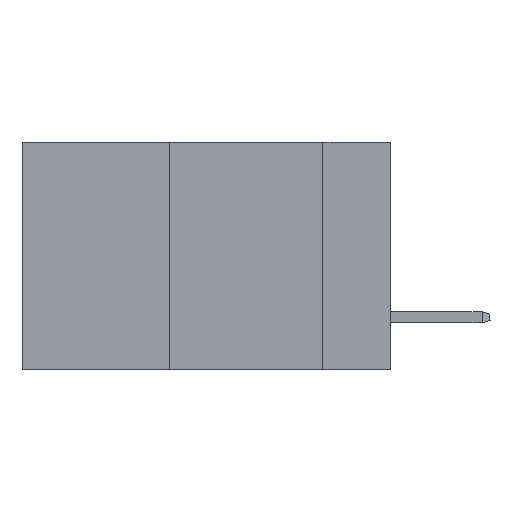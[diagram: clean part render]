
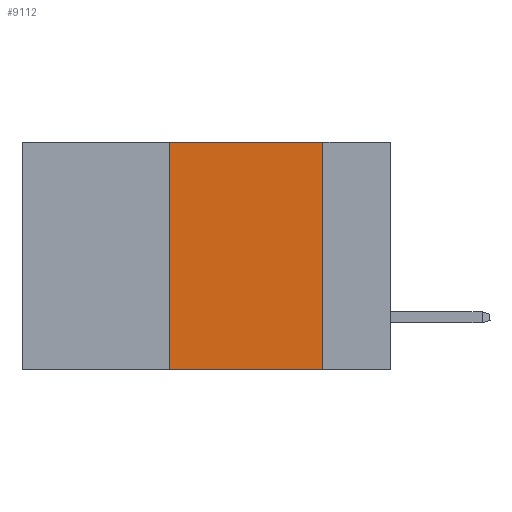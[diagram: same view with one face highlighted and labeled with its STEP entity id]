
A CAD part, left-side view. The second image highlights one B-rep face of the part: STEP entity #9112.
In plain terms, the highlighted planar face has unit normal (-1, 0, 0).
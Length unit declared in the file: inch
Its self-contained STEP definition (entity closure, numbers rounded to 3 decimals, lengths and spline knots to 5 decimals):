
#320 = CARTESIAN_POINT ( 'NONE',  ( 0., 0.11, -0.37 ) ) ;
#380 = CARTESIAN_POINT ( 'NONE',  ( 0., 0.6, -0.37 ) ) ;
#585 = ORIENTED_EDGE ( 'NONE', *, *, #3859, .F. ) ;
#831 = CARTESIAN_POINT ( 'NONE',  ( 0., 0.36, 0. ) ) ;
#1301 = EDGE_CURVE ( 'NONE', #4747, #1466, #3423, .T. ) ;
#1466 = VERTEX_POINT ( 'NONE', #320 ) ;
#3423 = LINE ( 'NONE', #7408, #4202 ) ;
#3859 = EDGE_CURVE ( 'NONE', #12912, #9530, #15747, .T. ) ;
#4006 = DIRECTION ( 'NONE',  ( 0., -1., 0. ) ) ;
#4202 = VECTOR ( 'NONE', #14901, 39.37008 ) ;
#4369 = AXIS2_PLACEMENT_3D ( 'NONE', #11024, #6179, #13706 ) ;
#4747 = VERTEX_POINT ( 'NONE', #6330 ) ;
#5674 = LINE ( 'NONE', #11417, #7056 ) ;
#5912 = LINE ( 'NONE', #380, #14829 ) ;
#6025 = VECTOR ( 'NONE', #6158, 39.37008 ) ;
#6158 = DIRECTION ( 'NONE',  ( 0., 0., 1. ) ) ;
#6179 = DIRECTION ( 'NONE',  ( 1., 0., 0. ) ) ;
#6330 = CARTESIAN_POINT ( 'NONE',  ( 0., 0.11, 0. ) ) ;
#6466 = ORIENTED_EDGE ( 'NONE', *, *, #1301, .F. ) ;
#7056 = VECTOR ( 'NONE', #4006, 39.37008 ) ;
#7227 = PLANE ( 'NONE',  #4369 ) ;
#7408 = CARTESIAN_POINT ( 'NONE',  ( 0., 0.11, 0. ) ) ;
#7423 = EDGE_CURVE ( 'NONE', #12912, #1466, #5912, .T. ) ;
#8384 = EDGE_CURVE ( 'NONE', #9530, #4747, #5674, .T. ) ;
#9112 = ADVANCED_FACE ( 'NONE', ( #10205 ), #7227, .F. ) ;
#9157 = ORIENTED_EDGE ( 'NONE', *, *, #7423, .T. ) ;
#9530 = VERTEX_POINT ( 'NONE', #831 ) ;
#10018 = CARTESIAN_POINT ( 'NONE',  ( 0., 0.36, 0. ) ) ;
#10147 = CARTESIAN_POINT ( 'NONE',  ( 0., 0.36, -0.37 ) ) ;
#10205 = FACE_OUTER_BOUND ( 'NONE', #14253, .T. ) ;
#10339 = DIRECTION ( 'NONE',  ( 0., -1., 0. ) ) ;
#11024 = CARTESIAN_POINT ( 'NONE',  ( 0., 0.6, 0. ) ) ;
#11417 = CARTESIAN_POINT ( 'NONE',  ( 0., 0.6, 0. ) ) ;
#11807 = ORIENTED_EDGE ( 'NONE', *, *, #8384, .F. ) ;
#12912 = VERTEX_POINT ( 'NONE', #10147 ) ;
#13706 = DIRECTION ( 'NONE',  ( 0., 0., -1. ) ) ;
#14253 = EDGE_LOOP ( 'NONE', ( #6466, #11807, #585, #9157 ) ) ;
#14829 = VECTOR ( 'NONE', #10339, 39.37008 ) ;
#14901 = DIRECTION ( 'NONE',  ( 0., 0., -1. ) ) ;
#15747 = LINE ( 'NONE', #10018, #6025 ) ;
